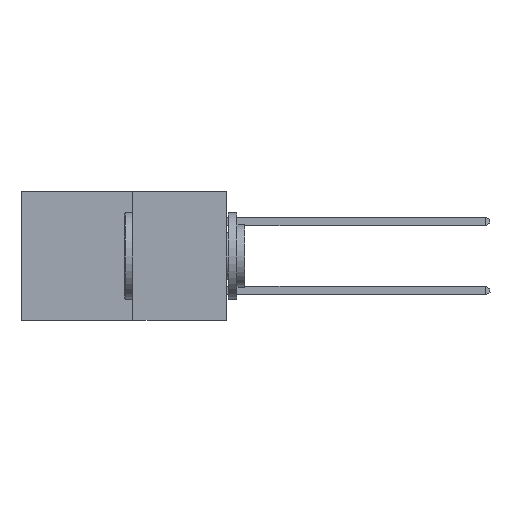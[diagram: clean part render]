
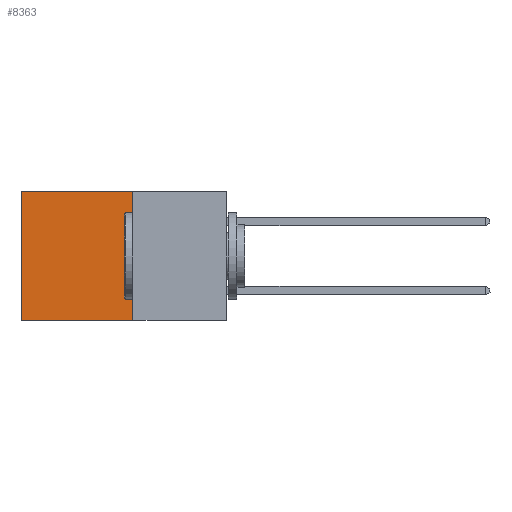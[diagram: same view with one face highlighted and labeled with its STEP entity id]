
A CAD part, left-side view. The second image highlights one B-rep face of the part: STEP entity #8363.
In plain terms, the highlighted planar face has unit normal (-1, 0, 0).
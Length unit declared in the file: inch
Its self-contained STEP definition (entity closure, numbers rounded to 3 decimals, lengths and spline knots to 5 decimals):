
#320 = FACE_OUTER_BOUND ( 'NONE', #9568, .T. ) ;
#1750 = VECTOR ( 'NONE', #20384, 39.37008 ) ;
#2539 = VECTOR ( 'NONE', #12669, 39.37008 ) ;
#3330 = EDGE_CURVE ( 'NONE', #3501, #6506, #14683, .T. ) ;
#3462 = DIRECTION ( 'NONE',  ( 0., 0., -1. ) ) ;
#3501 = VERTEX_POINT ( 'NONE', #20127 ) ;
#3655 = LINE ( 'NONE', #20546, #16606 ) ;
#4317 = PLANE ( 'NONE',  #14911 ) ;
#4334 = ORIENTED_EDGE ( 'NONE', *, *, #15259, .T. ) ;
#5670 = VECTOR ( 'NONE', #9135, 39.37008 ) ;
#6473 = EDGE_CURVE ( 'NONE', #9367, #6506, #14815, .T. ) ;
#6506 = VERTEX_POINT ( 'NONE', #13930 ) ;
#6814 = CARTESIAN_POINT ( 'NONE',  ( 0.277, 0.27, -0.37 ) ) ;
#7075 = LINE ( 'NONE', #20869, #2539 ) ;
#8363 = ADVANCED_FACE ( 'NONE', ( #320 ), #4317, .F. ) ;
#8734 = CARTESIAN_POINT ( 'NONE',  ( 0.277, 0.59, -0.37 ) ) ;
#9135 = DIRECTION ( 'NONE',  ( 0., 1., 0. ) ) ;
#9170 = VERTEX_POINT ( 'NONE', #16620 ) ;
#9367 = VERTEX_POINT ( 'NONE', #18710 ) ;
#9568 = EDGE_LOOP ( 'NONE', ( #14516, #14093, #14425, #4334 ) ) ;
#9860 = CARTESIAN_POINT ( 'NONE',  ( 0.277, 0.27, -0.37 ) ) ;
#12669 = DIRECTION ( 'NONE',  ( 0., 1., 0. ) ) ;
#12820 = EDGE_CURVE ( 'NONE', #9170, #3501, #3655, .T. ) ;
#13647 = DIRECTION ( 'NONE',  ( 1., 0., 0. ) ) ;
#13930 = CARTESIAN_POINT ( 'NONE',  ( 0.277, 0.59, -0.37 ) ) ;
#14093 = ORIENTED_EDGE ( 'NONE', *, *, #3330, .F. ) ;
#14425 = ORIENTED_EDGE ( 'NONE', *, *, #12820, .F. ) ;
#14516 = ORIENTED_EDGE ( 'NONE', *, *, #6473, .T. ) ;
#14683 = LINE ( 'NONE', #9860, #5670 ) ;
#14815 = LINE ( 'NONE', #8734, #1750 ) ;
#14911 = AXIS2_PLACEMENT_3D ( 'NONE', #6814, #13647, #3462 ) ;
#15259 = EDGE_CURVE ( 'NONE', #9170, #9367, #7075, .T. ) ;
#15652 = DIRECTION ( 'NONE',  ( 0., 0., -1. ) ) ;
#16606 = VECTOR ( 'NONE', #15652, 39.37008 ) ;
#16620 = CARTESIAN_POINT ( 'NONE',  ( 0.277, 0.27, 0. ) ) ;
#18710 = CARTESIAN_POINT ( 'NONE',  ( 0.277, 0.59, 0. ) ) ;
#20127 = CARTESIAN_POINT ( 'NONE',  ( 0.277, 0.27, -0.37 ) ) ;
#20384 = DIRECTION ( 'NONE',  ( 0., 0., -1. ) ) ;
#20546 = CARTESIAN_POINT ( 'NONE',  ( 0.277, 0.27, -0.37 ) ) ;
#20869 = CARTESIAN_POINT ( 'NONE',  ( 0.277, 0.27, 0. ) ) ;
